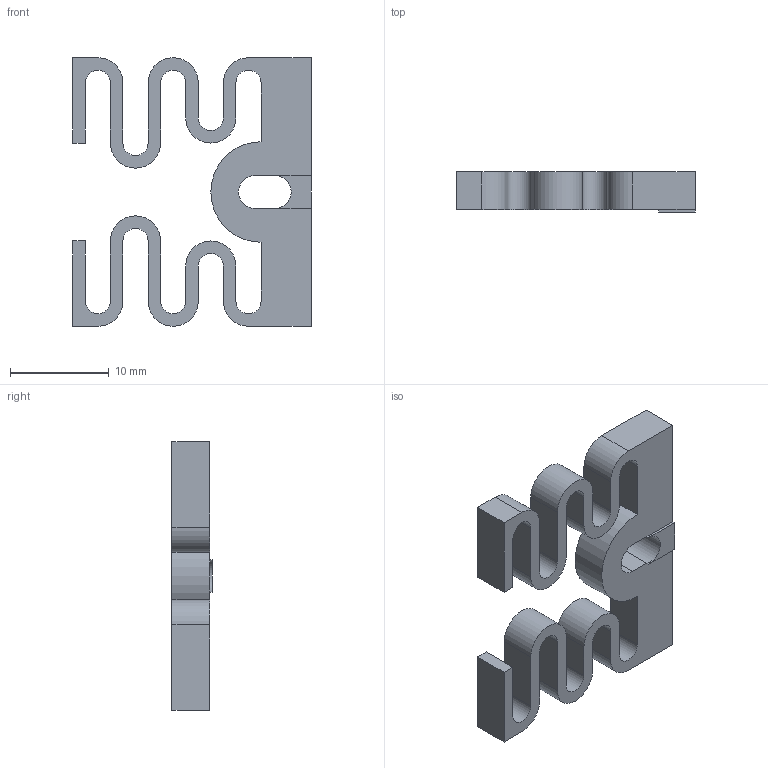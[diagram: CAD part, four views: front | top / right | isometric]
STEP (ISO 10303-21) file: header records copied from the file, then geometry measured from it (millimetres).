
FILE_DESCRIPTION (( 'STEP AP214' ), '1' );
FILE_NAME ('trigger_spring.STEP', '2013-06-07T17:14:41', ( 'Asher' ), ( '' ), 'SwSTEP 2.0', 'SolidWorks 2013', '' );
FILE_SCHEMA (( 'AUTOMOTIVE_DESIGN' ));
Length unit declared in the file: inch
Products named in the file (1): trigger_spring
Bounding box: 24.13 x 4.06 x 27.18 mm (x, y, z)
Volume: 1156.2 mm3; surface area: 1753.8 mm2
Topology: 1 solids, 1 shells, 59 faces, 172 edges, 114 vertices
Faces by surface type: plane 36, cylinder 23
Entity records: 2000 total; most frequent: CARTESIAN_POINT 346, ORIENTED_EDGE 344, DIRECTION 338, EDGE_CURVE 172, VECTOR 126, LINE 126, VERTEX_POINT 114, AXIS2_PLACEMENT_3D 106
